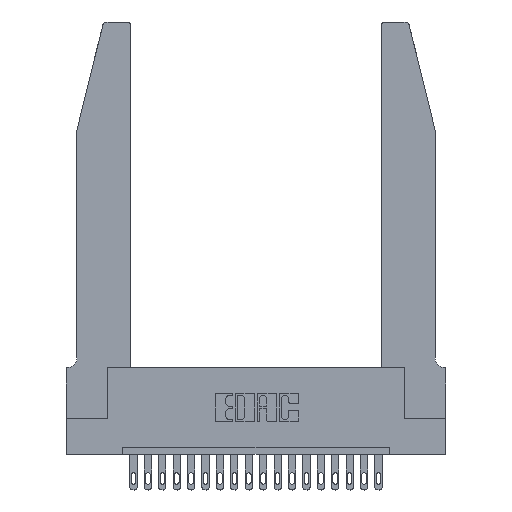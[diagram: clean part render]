
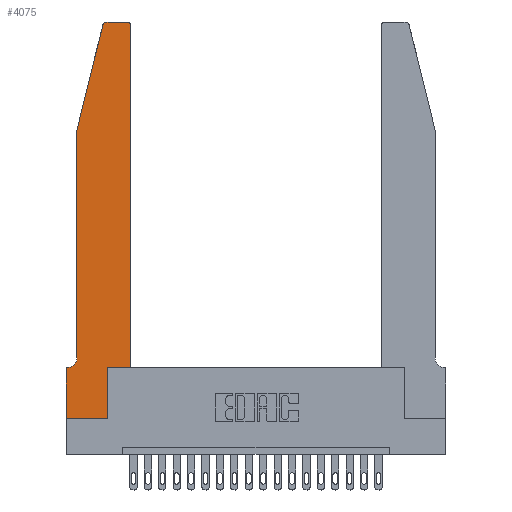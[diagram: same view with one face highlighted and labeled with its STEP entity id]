
A CAD part, top view. The second image highlights one B-rep face of the part: STEP entity #4075.
In plain terms, the highlighted planar face has unit normal (0, 0, 1).
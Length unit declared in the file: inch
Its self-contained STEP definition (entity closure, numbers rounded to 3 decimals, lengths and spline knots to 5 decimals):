
#36 = ORIENTED_EDGE ( 'NONE', *, *, #6200, .T. ) ;
#77 = LINE ( 'NONE', #5636, #7067 ) ;
#466 = EDGE_LOOP ( 'NONE', ( #9623, #5362, #36, #3382, #16817, #11190, #17186, #3431, #9653, #20507, #10497, #19729 ) ) ;
#589 = LINE ( 'NONE', #10998, #5262 ) ;
#741 = DIRECTION ( 'NONE',  ( 1., 0., 0. ) ) ;
#1141 = VECTOR ( 'NONE', #19944, 39.37008 ) ;
#1656 = LINE ( 'NONE', #11361, #1141 ) ;
#2071 = VERTEX_POINT ( 'NONE', #13715 ) ;
#2229 = LINE ( 'NONE', #18465, #20352 ) ;
#2373 = LINE ( 'NONE', #5974, #8307 ) ;
#2605 = AXIS2_PLACEMENT_3D ( 'NONE', #7525, #14250, #741 ) ;
#2747 = VECTOR ( 'NONE', #16583, 39.37008 ) ;
#3048 = CARTESIAN_POINT ( 'NONE',  ( 0.2865, 0.35, 0.37 ) ) ;
#3069 = VERTEX_POINT ( 'NONE', #20662 ) ;
#3163 = CIRCLE ( 'NONE', #2605, 0.03 ) ;
#3184 = AXIS2_PLACEMENT_3D ( 'NONE', #10596, #7189, #10522 ) ;
#3348 = CARTESIAN_POINT ( 'NONE',  ( 0.284, 2.72, 0.37 ) ) ;
#3382 = ORIENTED_EDGE ( 'NONE', *, *, #21291, .T. ) ;
#3431 = ORIENTED_EDGE ( 'NONE', *, *, #13602, .T. ) ;
#3967 = LINE ( 'NONE', #10397, #20534 ) ;
#3977 = DIRECTION ( 'NONE',  ( 0., -1., 0. ) ) ;
#4075 = ADVANCED_FACE ( 'NONE', ( #15642 ), #14934, .T. ) ;
#5027 = DIRECTION ( 'NONE',  ( 1., 0., 0. ) ) ;
#5262 = VECTOR ( 'NONE', #16162, 39.37008 ) ;
#5362 = ORIENTED_EDGE ( 'NONE', *, *, #20435, .T. ) ;
#5523 = VERTEX_POINT ( 'NONE', #5772 ) ;
#5570 = LINE ( 'NONE', #18210, #17987 ) ;
#5595 = EDGE_CURVE ( 'NONE', #6275, #5523, #5866, .T. ) ;
#5636 = CARTESIAN_POINT ( 'NONE',  ( 0.0755, 0.35, 0.37 ) ) ;
#5772 = CARTESIAN_POINT ( 'NONE',  ( 0.2865, 0.35, 0.37 ) ) ;
#5866 = LINE ( 'NONE', #3048, #2747 ) ;
#5974 = CARTESIAN_POINT ( 'NONE',  ( 0.4505, 0.35, 0.37 ) ) ;
#6200 = EDGE_CURVE ( 'NONE', #19092, #15062, #5570, .T. ) ;
#6275 = VERTEX_POINT ( 'NONE', #18969 ) ;
#6631 = DIRECTION ( 'NONE',  ( 1., 0., 0. ) ) ;
#7067 = VECTOR ( 'NONE', #17427, 39.37008 ) ;
#7189 = DIRECTION ( 'NONE',  ( 0., 0., -1. ) ) ;
#7525 = CARTESIAN_POINT ( 'NONE',  ( 0.4205, 2.72, 0.37 ) ) ;
#8062 = VERTEX_POINT ( 'NONE', #18216 ) ;
#8149 = VERTEX_POINT ( 'NONE', #11491 ) ;
#8307 = VECTOR ( 'NONE', #19284, 39.37008 ) ;
#8510 = VECTOR ( 'NONE', #20479, 39.37008 ) ;
#9030 = LINE ( 'NONE', #13785, #8510 ) ;
#9093 = EDGE_CURVE ( 'NONE', #14277, #3069, #9030, .T. ) ;
#9194 = CARTESIAN_POINT ( 'NONE',  ( 0.4505, 0.35, 0.37 ) ) ;
#9623 = ORIENTED_EDGE ( 'NONE', *, *, #13939, .T. ) ;
#9653 = ORIENTED_EDGE ( 'NONE', *, *, #5595, .T. ) ;
#10047 = CARTESIAN_POINT ( 'NONE',  ( 0., 0.35, 0.37 ) ) ;
#10397 = CARTESIAN_POINT ( 'NONE',  ( 0.0755, 2., 0.37 ) ) ;
#10497 = ORIENTED_EDGE ( 'NONE', *, *, #10994, .T. ) ;
#10522 = DIRECTION ( 'NONE',  ( -1., 0., 0. ) ) ;
#10541 = VERTEX_POINT ( 'NONE', #9194 ) ;
#10596 = CARTESIAN_POINT ( 'NONE',  ( 0.0055, 0.42, 0.37 ) ) ;
#10994 = EDGE_CURVE ( 'NONE', #10541, #2071, #2229, .T. ) ;
#10998 = CARTESIAN_POINT ( 'NONE',  ( 0.2605, 2.75, 0.37 ) ) ;
#11190 = ORIENTED_EDGE ( 'NONE', *, *, #19695, .T. ) ;
#11361 = CARTESIAN_POINT ( 'NONE',  ( 0., 0., 0.37 ) ) ;
#11491 = CARTESIAN_POINT ( 'NONE',  ( 0.0755, 0.42, 0.37 ) ) ;
#11935 = CIRCLE ( 'NONE', #16743, 0.03 ) ;
#12266 = EDGE_CURVE ( 'NONE', #8149, #13161, #15436, .T. ) ;
#12471 = CARTESIAN_POINT ( 'NONE',  ( 0.284, 2.75, 0.37 ) ) ;
#13152 = CARTESIAN_POINT ( 'NONE',  ( 0., 0.35, 0.37 ) ) ;
#13161 = VERTEX_POINT ( 'NONE', #18107 ) ;
#13602 = EDGE_CURVE ( 'NONE', #3069, #6275, #1656, .T. ) ;
#13715 = CARTESIAN_POINT ( 'NONE',  ( 0.4505, 2.72, 0.37 ) ) ;
#13785 = CARTESIAN_POINT ( 'NONE',  ( 0., 0., 0.37 ) ) ;
#13939 = EDGE_CURVE ( 'NONE', #8062, #19188, #589, .T. ) ;
#14250 = DIRECTION ( 'NONE',  ( 0., 0., 1. ) ) ;
#14277 = VERTEX_POINT ( 'NONE', #10047 ) ;
#14829 = AXIS2_PLACEMENT_3D ( 'NONE', #13152, #14863, #6631 ) ;
#14863 = DIRECTION ( 'NONE',  ( 0., 0., 1. ) ) ;
#14934 = PLANE ( 'NONE',  #14829 ) ;
#15062 = VERTEX_POINT ( 'NONE', #20764 ) ;
#15129 = DIRECTION ( 'NONE',  ( 0., 0., 1. ) ) ;
#15436 = CIRCLE ( 'NONE', #3184, 0.07 ) ;
#15491 = EDGE_CURVE ( 'NONE', #5523, #10541, #2373, .T. ) ;
#15642 = FACE_OUTER_BOUND ( 'NONE', #466, .T. ) ;
#16162 = DIRECTION ( 'NONE',  ( -1., 0., 0. ) ) ;
#16583 = DIRECTION ( 'NONE',  ( 0., 1., 0. ) ) ;
#16743 = AXIS2_PLACEMENT_3D ( 'NONE', #3348, #15129, #5027 ) ;
#16817 = ORIENTED_EDGE ( 'NONE', *, *, #12266, .T. ) ;
#17186 = ORIENTED_EDGE ( 'NONE', *, *, #9093, .T. ) ;
#17427 = DIRECTION ( 'NONE',  ( -1., 0., 0. ) ) ;
#17987 = VECTOR ( 'NONE', #19778, 39.37008 ) ;
#18107 = CARTESIAN_POINT ( 'NONE',  ( 0.0055, 0.35, 0.37 ) ) ;
#18210 = CARTESIAN_POINT ( 'NONE',  ( 0.0755, 2., 0.37 ) ) ;
#18216 = CARTESIAN_POINT ( 'NONE',  ( 0.4205, 2.75, 0.37 ) ) ;
#18465 = CARTESIAN_POINT ( 'NONE',  ( 0.4505, 0.35, 0.37 ) ) ;
#18537 = DIRECTION ( 'NONE',  ( 0., 1., 0. ) ) ;
#18969 = CARTESIAN_POINT ( 'NONE',  ( 0.2865, 0., 0.37 ) ) ;
#19092 = VERTEX_POINT ( 'NONE', #20711 ) ;
#19188 = VERTEX_POINT ( 'NONE', #12471 ) ;
#19284 = DIRECTION ( 'NONE',  ( 1., 0., 0. ) ) ;
#19695 = EDGE_CURVE ( 'NONE', #13161, #14277, #77, .T. ) ;
#19729 = ORIENTED_EDGE ( 'NONE', *, *, #20756, .T. ) ;
#19778 = DIRECTION ( 'NONE',  ( -0.239, -0.971, 0. ) ) ;
#19944 = DIRECTION ( 'NONE',  ( 1., 0., 0. ) ) ;
#20352 = VECTOR ( 'NONE', #18537, 39.37008 ) ;
#20435 = EDGE_CURVE ( 'NONE', #19188, #19092, #11935, .T. ) ;
#20479 = DIRECTION ( 'NONE',  ( 0., -1., 0. ) ) ;
#20507 = ORIENTED_EDGE ( 'NONE', *, *, #15491, .T. ) ;
#20534 = VECTOR ( 'NONE', #3977, 39.37008 ) ;
#20662 = CARTESIAN_POINT ( 'NONE',  ( 0., 0., 0.37 ) ) ;
#20711 = CARTESIAN_POINT ( 'NONE',  ( 0.25487, 2.72718, 0.37 ) ) ;
#20756 = EDGE_CURVE ( 'NONE', #2071, #8062, #3163, .T. ) ;
#20764 = CARTESIAN_POINT ( 'NONE',  ( 0.0755, 2., 0.37 ) ) ;
#21291 = EDGE_CURVE ( 'NONE', #15062, #8149, #3967, .T. ) ;
